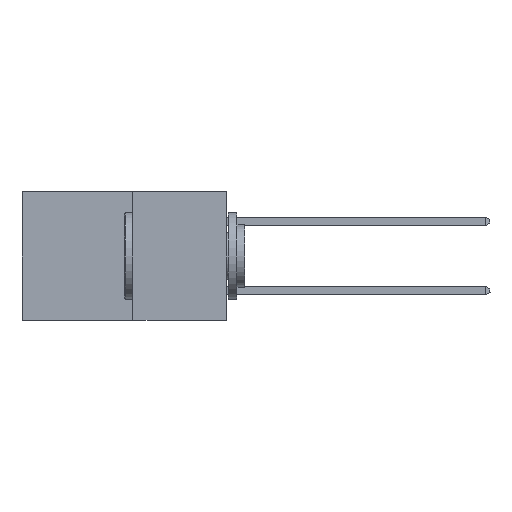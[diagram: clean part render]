
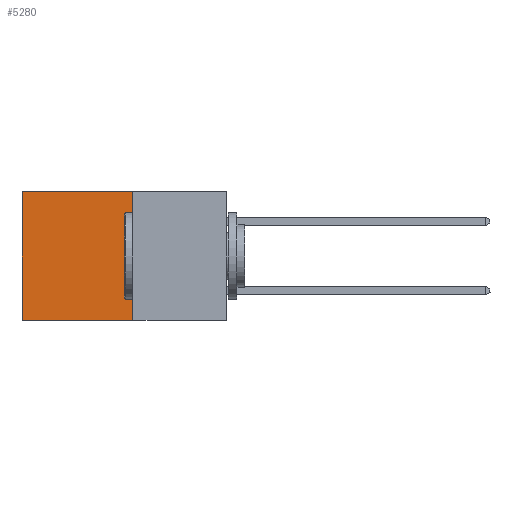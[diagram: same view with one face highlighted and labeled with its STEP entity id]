
A CAD part, left-side view. The second image highlights one B-rep face of the part: STEP entity #5280.
In plain terms, the highlighted planar face has unit normal (-1, 0, 0).
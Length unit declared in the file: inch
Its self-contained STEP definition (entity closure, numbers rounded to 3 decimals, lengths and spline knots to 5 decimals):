
#642 = CARTESIAN_POINT ( 'NONE',  ( 0.277, 0.59, -0.37 ) ) ;
#1508 = CARTESIAN_POINT ( 'NONE',  ( 0.277, 0.27, -0.37 ) ) ;
#1552 = LINE ( 'NONE', #1508, #2801 ) ;
#1715 = DIRECTION ( 'NONE',  ( 1., 0., 0. ) ) ;
#1949 = VECTOR ( 'NONE', #16286, 39.37008 ) ;
#2801 = VECTOR ( 'NONE', #15419, 39.37008 ) ;
#3955 = CARTESIAN_POINT ( 'NONE',  ( 0.277, 0.27, -0.37 ) ) ;
#3997 = EDGE_CURVE ( 'NONE', #21295, #5311, #11020, .T. ) ;
#4154 = DIRECTION ( 'NONE',  ( 0., 0., -1. ) ) ;
#5280 = ADVANCED_FACE ( 'NONE', ( #14035 ), #9768, .F. ) ;
#5311 = VERTEX_POINT ( 'NONE', #20186 ) ;
#6325 = VECTOR ( 'NONE', #13623, 39.37008 ) ;
#7272 = LINE ( 'NONE', #18148, #1949 ) ;
#8599 = AXIS2_PLACEMENT_3D ( 'NONE', #17485, #1715, #4154 ) ;
#8985 = VECTOR ( 'NONE', #10586, 39.37008 ) ;
#9768 = PLANE ( 'NONE',  #8599 ) ;
#10586 = DIRECTION ( 'NONE',  ( 0., 0., -1. ) ) ;
#11020 = LINE ( 'NONE', #3955, #6325 ) ;
#11225 = ORIENTED_EDGE ( 'NONE', *, *, #14376, .T. ) ;
#12024 = EDGE_CURVE ( 'NONE', #5311, #19438, #1552, .T. ) ;
#12420 = ORIENTED_EDGE ( 'NONE', *, *, #12024, .F. ) ;
#13623 = DIRECTION ( 'NONE',  ( 0., 0., -1. ) ) ;
#13675 = VERTEX_POINT ( 'NONE', #18178 ) ;
#13977 = ORIENTED_EDGE ( 'NONE', *, *, #3997, .F. ) ;
#14035 = FACE_OUTER_BOUND ( 'NONE', #14092, .T. ) ;
#14092 = EDGE_LOOP ( 'NONE', ( #19691, #12420, #13977, #11225 ) ) ;
#14376 = EDGE_CURVE ( 'NONE', #21295, #13675, #7272, .T. ) ;
#15419 = DIRECTION ( 'NONE',  ( 0., 1., 0. ) ) ;
#16286 = DIRECTION ( 'NONE',  ( 0., 1., 0. ) ) ;
#16708 = CARTESIAN_POINT ( 'NONE',  ( 0.277, 0.59, -0.37 ) ) ;
#17485 = CARTESIAN_POINT ( 'NONE',  ( 0.277, 0.27, -0.37 ) ) ;
#18148 = CARTESIAN_POINT ( 'NONE',  ( 0.277, 0.27, 0. ) ) ;
#18178 = CARTESIAN_POINT ( 'NONE',  ( 0.277, 0.59, 0. ) ) ;
#19438 = VERTEX_POINT ( 'NONE', #16708 ) ;
#19691 = ORIENTED_EDGE ( 'NONE', *, *, #24147, .T. ) ;
#20030 = CARTESIAN_POINT ( 'NONE',  ( 0.277, 0.27, 0. ) ) ;
#20186 = CARTESIAN_POINT ( 'NONE',  ( 0.277, 0.27, -0.37 ) ) ;
#21295 = VERTEX_POINT ( 'NONE', #20030 ) ;
#24147 = EDGE_CURVE ( 'NONE', #13675, #19438, #25233, .T. ) ;
#25233 = LINE ( 'NONE', #642, #8985 ) ;
